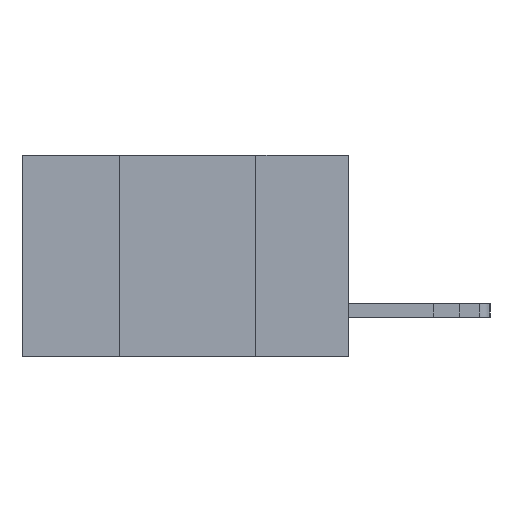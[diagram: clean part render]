
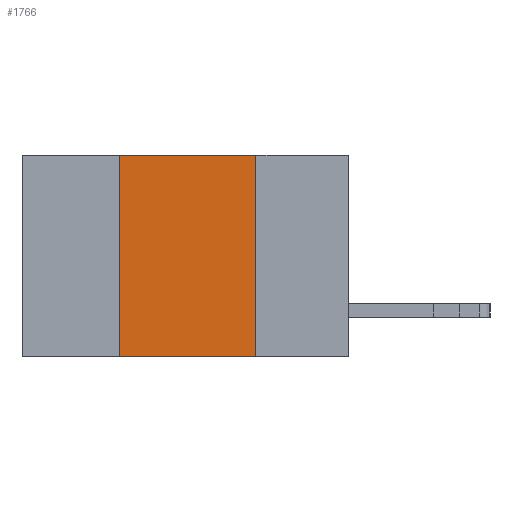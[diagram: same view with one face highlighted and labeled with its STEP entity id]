
A CAD part, left-side view. The second image highlights one B-rep face of the part: STEP entity #1766.
In plain terms, the highlighted planar face has unit normal (-1, 0, 0).
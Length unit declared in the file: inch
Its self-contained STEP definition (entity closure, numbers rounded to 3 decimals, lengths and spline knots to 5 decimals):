
#102 = VECTOR ( 'NONE', #6418, 39.37008 ) ;
#265 = VECTOR ( 'NONE', #7557, 39.37008 ) ;
#541 = CARTESIAN_POINT ( 'NONE',  ( 0., 0.17, -0.37 ) ) ;
#589 = VECTOR ( 'NONE', #4314, 39.37008 ) ;
#783 = AXIS2_PLACEMENT_3D ( 'NONE', #11488, #6820, #6554 ) ;
#984 = CARTESIAN_POINT ( 'NONE',  ( 0., 0.17, 0. ) ) ;
#1109 = LINE ( 'NONE', #6302, #265 ) ;
#1224 = EDGE_CURVE ( 'NONE', #6989, #3802, #6917, .T. ) ;
#1766 = ADVANCED_FACE ( 'NONE', ( #7915 ), #7558, .F. ) ;
#2194 = EDGE_LOOP ( 'NONE', ( #9912, #5138, #10317, #3210 ) ) ;
#2362 = CARTESIAN_POINT ( 'NONE',  ( 0., 0.6, 0. ) ) ;
#3210 = ORIENTED_EDGE ( 'NONE', *, *, #1224, .T. ) ;
#3802 = VERTEX_POINT ( 'NONE', #541 ) ;
#4063 = EDGE_CURVE ( 'NONE', #16813, #9349, #14218, .T. ) ;
#4314 = DIRECTION ( 'NONE',  ( 0., 0., 1. ) ) ;
#5138 = ORIENTED_EDGE ( 'NONE', *, *, #4063, .F. ) ;
#5766 = EDGE_CURVE ( 'NONE', #6989, #16813, #7712, .T. ) ;
#6302 = CARTESIAN_POINT ( 'NONE',  ( 0., 0.17, 0. ) ) ;
#6418 = DIRECTION ( 'NONE',  ( 0., -1., 0. ) ) ;
#6502 = VECTOR ( 'NONE', #10216, 39.37008 ) ;
#6554 = DIRECTION ( 'NONE',  ( 0., 0., -1. ) ) ;
#6820 = DIRECTION ( 'NONE',  ( 1., 0., 0. ) ) ;
#6900 = CARTESIAN_POINT ( 'NONE',  ( 0., 0.42, -0.37 ) ) ;
#6917 = LINE ( 'NONE', #11041, #6502 ) ;
#6989 = VERTEX_POINT ( 'NONE', #6900 ) ;
#7557 = DIRECTION ( 'NONE',  ( 0., 0., -1. ) ) ;
#7558 = PLANE ( 'NONE',  #783 ) ;
#7712 = LINE ( 'NONE', #11002, #589 ) ;
#7915 = FACE_OUTER_BOUND ( 'NONE', #2194, .T. ) ;
#9318 = EDGE_CURVE ( 'NONE', #9349, #3802, #1109, .T. ) ;
#9349 = VERTEX_POINT ( 'NONE', #984 ) ;
#9912 = ORIENTED_EDGE ( 'NONE', *, *, #9318, .F. ) ;
#10216 = DIRECTION ( 'NONE',  ( 0., -1., 0. ) ) ;
#10317 = ORIENTED_EDGE ( 'NONE', *, *, #5766, .F. ) ;
#11002 = CARTESIAN_POINT ( 'NONE',  ( 0., 0.42, 0. ) ) ;
#11041 = CARTESIAN_POINT ( 'NONE',  ( 0., 0.6, -0.37 ) ) ;
#11488 = CARTESIAN_POINT ( 'NONE',  ( 0., 0.6, 0. ) ) ;
#14218 = LINE ( 'NONE', #2362, #102 ) ;
#16813 = VERTEX_POINT ( 'NONE', #16924 ) ;
#16924 = CARTESIAN_POINT ( 'NONE',  ( 0., 0.42, 0. ) ) ;
